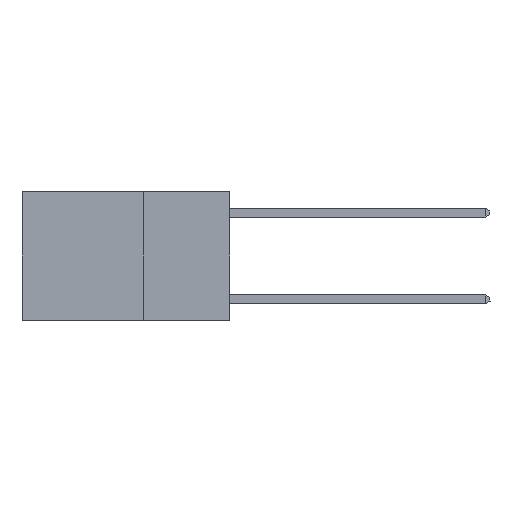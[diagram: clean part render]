
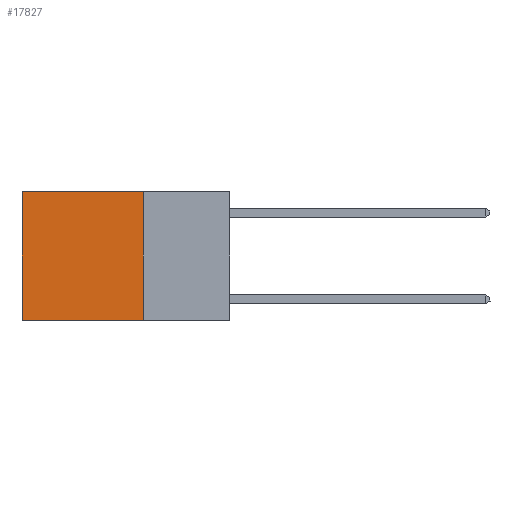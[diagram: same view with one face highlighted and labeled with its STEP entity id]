
A CAD part, left-side view. The second image highlights one B-rep face of the part: STEP entity #17827.
In plain terms, the highlighted planar face has unit normal (-1, 0, 0).
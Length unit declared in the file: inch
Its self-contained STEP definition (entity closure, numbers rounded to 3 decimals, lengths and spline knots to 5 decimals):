
#372 = ORIENTED_EDGE ( 'NONE', *, *, #6387, .F. ) ;
#1454 = CARTESIAN_POINT ( 'NONE',  ( 0.2625, 0.6, 0. ) ) ;
#2508 = PLANE ( 'NONE',  #3426 ) ;
#3041 = LINE ( 'NONE', #3445, #15470 ) ;
#3426 = AXIS2_PLACEMENT_3D ( 'NONE', #14373, #16026, #17768 ) ;
#3445 = CARTESIAN_POINT ( 'NONE',  ( 0.2625, 0.25, 0. ) ) ;
#3721 = EDGE_CURVE ( 'NONE', #10729, #14600, #13588, .T. ) ;
#3871 = CARTESIAN_POINT ( 'NONE',  ( 0.2625, 0.25, -0.37 ) ) ;
#6387 = EDGE_CURVE ( 'NONE', #21229, #7429, #15334, .T. ) ;
#6644 = EDGE_CURVE ( 'NONE', #7429, #14600, #21484, .T. ) ;
#6755 = DIRECTION ( 'NONE',  ( 0., 1., 0. ) ) ;
#7429 = VERTEX_POINT ( 'NONE', #14142 ) ;
#7464 = FACE_OUTER_BOUND ( 'NONE', #9272, .T. ) ;
#8115 = CARTESIAN_POINT ( 'NONE',  ( 0.2625, 0.6, 0. ) ) ;
#9272 = EDGE_LOOP ( 'NONE', ( #15338, #20642, #372, #11115 ) ) ;
#9856 = DIRECTION ( 'NONE',  ( 0., 0., -1. ) ) ;
#10281 = VECTOR ( 'NONE', #9856, 39.37008 ) ;
#10569 = VECTOR ( 'NONE', #14031, 39.37008 ) ;
#10729 = VERTEX_POINT ( 'NONE', #8115 ) ;
#11115 = ORIENTED_EDGE ( 'NONE', *, *, #20545, .T. ) ;
#12843 = CARTESIAN_POINT ( 'NONE',  ( 0.2625, 0.25, 0. ) ) ;
#13277 = CARTESIAN_POINT ( 'NONE',  ( 0.2625, 0.6, -0.37 ) ) ;
#13588 = LINE ( 'NONE', #1454, #19684 ) ;
#14031 = DIRECTION ( 'NONE',  ( 0., 1., 0. ) ) ;
#14142 = CARTESIAN_POINT ( 'NONE',  ( 0.2625, 0.25, -0.37 ) ) ;
#14373 = CARTESIAN_POINT ( 'NONE',  ( 0.2625, 0.25, 0. ) ) ;
#14600 = VERTEX_POINT ( 'NONE', #13277 ) ;
#15334 = LINE ( 'NONE', #19884, #10281 ) ;
#15338 = ORIENTED_EDGE ( 'NONE', *, *, #3721, .T. ) ;
#15470 = VECTOR ( 'NONE', #6755, 39.37008 ) ;
#16026 = DIRECTION ( 'NONE',  ( 1., 0., 0. ) ) ;
#16540 = DIRECTION ( 'NONE',  ( 0., 0., -1. ) ) ;
#17768 = DIRECTION ( 'NONE',  ( 0., 0., -1. ) ) ;
#17827 = ADVANCED_FACE ( 'NONE', ( #7464 ), #2508, .F. ) ;
#19684 = VECTOR ( 'NONE', #16540, 39.37008 ) ;
#19884 = CARTESIAN_POINT ( 'NONE',  ( 0.2625, 0.25, 0. ) ) ;
#20545 = EDGE_CURVE ( 'NONE', #21229, #10729, #3041, .T. ) ;
#20642 = ORIENTED_EDGE ( 'NONE', *, *, #6644, .F. ) ;
#21229 = VERTEX_POINT ( 'NONE', #12843 ) ;
#21484 = LINE ( 'NONE', #3871, #10569 ) ;
